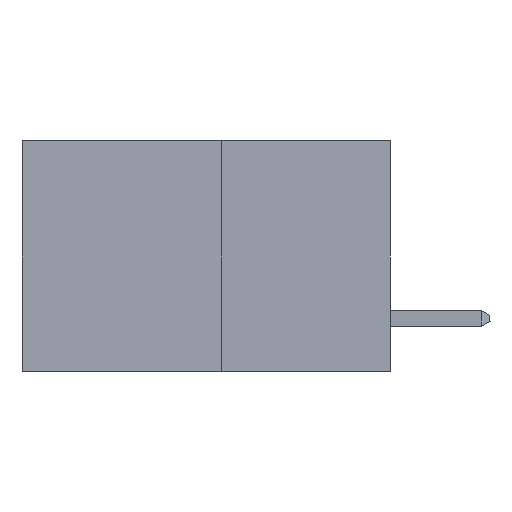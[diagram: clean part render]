
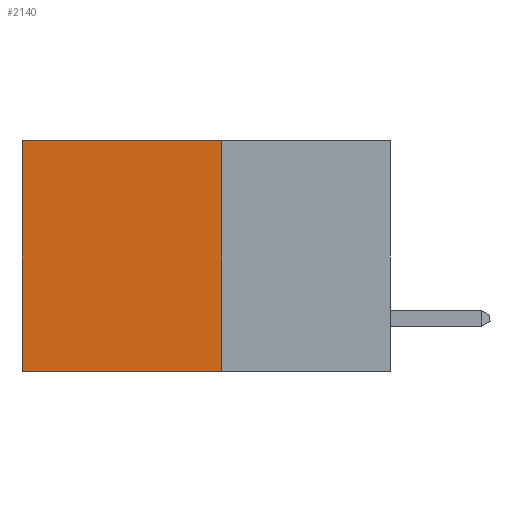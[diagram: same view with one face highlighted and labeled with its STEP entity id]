
A CAD part, left-side view. The second image highlights one B-rep face of the part: STEP entity #2140.
In plain terms, the highlighted planar face has unit normal (-1, 0, 0).
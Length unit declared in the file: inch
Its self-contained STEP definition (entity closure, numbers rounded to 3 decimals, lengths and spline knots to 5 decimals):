
#495 = LINE ( 'NONE', #12072, #10803 ) ;
#822 = EDGE_CURVE ( 'NONE', #13017, #17159, #10443, .T. ) ;
#1509 = VECTOR ( 'NONE', #21520, 39.37008 ) ;
#2025 = DIRECTION ( 'NONE',  ( 1., 0., 0. ) ) ;
#2061 = PLANE ( 'NONE',  #14891 ) ;
#2140 = ADVANCED_FACE ( 'NONE', ( #21093 ), #2061, .F. ) ;
#3734 = EDGE_LOOP ( 'NONE', ( #25544, #15944, #12538, #6899 ) ) ;
#4146 = LINE ( 'NONE', #22625, #24886 ) ;
#5398 = CARTESIAN_POINT ( 'NONE',  ( 0.277, 0.59, -0.37 ) ) ;
#6103 = DIRECTION ( 'NONE',  ( 0., 0., -1. ) ) ;
#6382 = VECTOR ( 'NONE', #10498, 39.37008 ) ;
#6782 = CARTESIAN_POINT ( 'NONE',  ( 0.277, 0.27, -0.37 ) ) ;
#6899 = ORIENTED_EDGE ( 'NONE', *, *, #17045, .T. ) ;
#10443 = LINE ( 'NONE', #6782, #6382 ) ;
#10498 = DIRECTION ( 'NONE',  ( 0., 1., 0. ) ) ;
#10500 = CARTESIAN_POINT ( 'NONE',  ( 0.277, 0.27, 0. ) ) ;
#10579 = DIRECTION ( 'NONE',  ( 0., 1., 0. ) ) ;
#10803 = VECTOR ( 'NONE', #6103, 39.37008 ) ;
#11000 = CARTESIAN_POINT ( 'NONE',  ( 0.277, 0.59, -0.37 ) ) ;
#12072 = CARTESIAN_POINT ( 'NONE',  ( 0.277, 0.27, -0.37 ) ) ;
#12538 = ORIENTED_EDGE ( 'NONE', *, *, #17443, .F. ) ;
#13017 = VERTEX_POINT ( 'NONE', #16222 ) ;
#14891 = AXIS2_PLACEMENT_3D ( 'NONE', #25183, #2025, #25037 ) ;
#15944 = ORIENTED_EDGE ( 'NONE', *, *, #822, .F. ) ;
#16222 = CARTESIAN_POINT ( 'NONE',  ( 0.277, 0.27, -0.37 ) ) ;
#17045 = EDGE_CURVE ( 'NONE', #17842, #21256, #4146, .T. ) ;
#17159 = VERTEX_POINT ( 'NONE', #11000 ) ;
#17176 = EDGE_CURVE ( 'NONE', #21256, #17159, #23070, .T. ) ;
#17443 = EDGE_CURVE ( 'NONE', #17842, #13017, #495, .T. ) ;
#17842 = VERTEX_POINT ( 'NONE', #10500 ) ;
#21093 = FACE_OUTER_BOUND ( 'NONE', #3734, .T. ) ;
#21256 = VERTEX_POINT ( 'NONE', #22745 ) ;
#21520 = DIRECTION ( 'NONE',  ( 0., 0., -1. ) ) ;
#22625 = CARTESIAN_POINT ( 'NONE',  ( 0.277, 0.27, 0. ) ) ;
#22745 = CARTESIAN_POINT ( 'NONE',  ( 0.277, 0.59, 0. ) ) ;
#23070 = LINE ( 'NONE', #5398, #1509 ) ;
#24886 = VECTOR ( 'NONE', #10579, 39.37008 ) ;
#25037 = DIRECTION ( 'NONE',  ( 0., 0., -1. ) ) ;
#25183 = CARTESIAN_POINT ( 'NONE',  ( 0.277, 0.27, -0.37 ) ) ;
#25544 = ORIENTED_EDGE ( 'NONE', *, *, #17176, .T. ) ;
